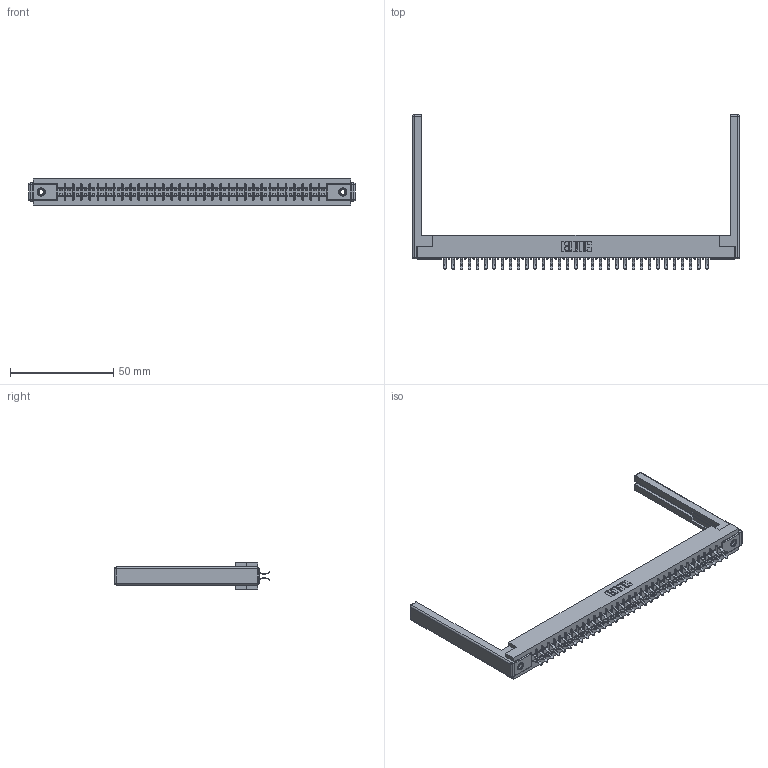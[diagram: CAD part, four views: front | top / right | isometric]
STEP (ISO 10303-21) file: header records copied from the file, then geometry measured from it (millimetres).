
FILE_DESCRIPTION (( 'STEP AP203' ), '1' );
FILE_NAME ('305-066-556-268.STEP', '2019-09-10T03:55:03', ( '' ), ( '' ), 'SwSTEP 2.0', 'SolidWorks 2016', '' );
FILE_SCHEMA (( 'CONFIG_CONTROL_DESIGN' ));
Length unit declared in the file: inch
Products named in the file (5): 305 Part_.156 Dia; 307-220-068; 305-066-556-268; 305-290-001_556; 345-250-001_345-250-001-102
Assembly tree (71 placements, depth 2):
  305-066-556-268
    305 Part_.156 Dia
    305-290-001_556  x66
    345-250-001_345-250-001-102  x2
    307-220-068  x2
Bounding box: 158.19 x 74.93 x 12.7 mm (x, y, z)
Volume: 20823.8 mm3; surface area: 24703.4 mm2
Topology: 71 solids, 71 shells, 3966 faces, 11365 edges, 7378 vertices
Faces by surface type: plane 2202, cylinder 1608, sphere 140, cone 12, torus 4
Entity records: 39807 total; most frequent: CARTESIAN_POINT 6562, ORIENTED_EDGE 6504, DIRECTION 6378, EDGE_CURVE 3252, LINE 2606, VECTOR 2606, VERTEX_POINT 2070, AXIS2_PLACEMENT_3D 1886
